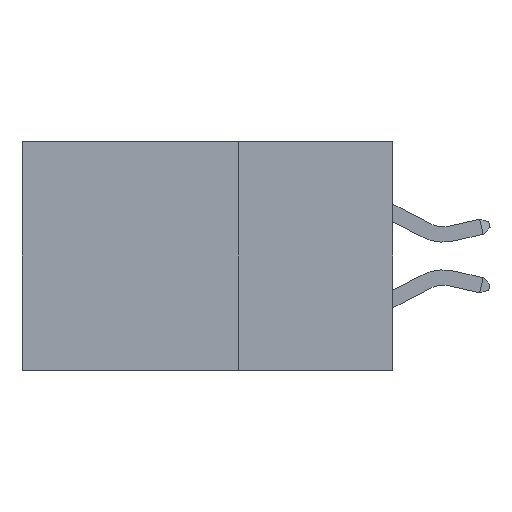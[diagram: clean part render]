
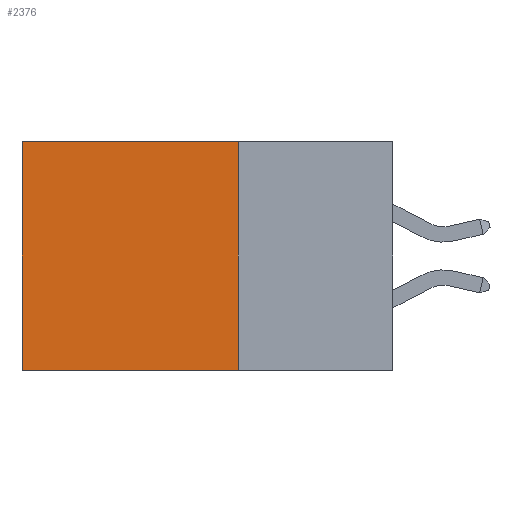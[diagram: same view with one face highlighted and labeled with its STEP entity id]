
A CAD part, left-side view. The second image highlights one B-rep face of the part: STEP entity #2376.
In plain terms, the highlighted planar face has unit normal (-1, 0, 0).
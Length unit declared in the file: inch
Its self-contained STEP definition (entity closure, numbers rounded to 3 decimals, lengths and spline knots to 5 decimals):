
#476 = VERTEX_POINT ( 'NONE', #19869 ) ;
#1830 = EDGE_CURVE ( 'NONE', #19514, #10616, #15404, .T. ) ;
#2038 = AXIS2_PLACEMENT_3D ( 'NONE', #9640, #19186, #17297 ) ;
#2376 = ADVANCED_FACE ( 'NONE', ( #4678 ), #13241, .F. ) ;
#2590 = ORIENTED_EDGE ( 'NONE', *, *, #21631, .T. ) ;
#2785 = CARTESIAN_POINT ( 'NONE',  ( 0.2875, 0.25, 0. ) ) ;
#2989 = CARTESIAN_POINT ( 'NONE',  ( 0.2875, 0.25, 0. ) ) ;
#4678 = FACE_OUTER_BOUND ( 'NONE', #10121, .T. ) ;
#5026 = VERTEX_POINT ( 'NONE', #10956 ) ;
#7851 = DIRECTION ( 'NONE',  ( 0., 1., 0. ) ) ;
#8581 = DIRECTION ( 'NONE',  ( 0., 0., -1. ) ) ;
#9120 = CARTESIAN_POINT ( 'NONE',  ( 0.2875, 0.25, -0.37 ) ) ;
#9324 = LINE ( 'NONE', #9120, #21638 ) ;
#9455 = EDGE_CURVE ( 'NONE', #10616, #476, #9324, .T. ) ;
#9640 = CARTESIAN_POINT ( 'NONE',  ( 0.2875, 0.25, 0. ) ) ;
#10121 = EDGE_LOOP ( 'NONE', ( #19588, #12713, #20958, #2590 ) ) ;
#10182 = CARTESIAN_POINT ( 'NONE',  ( 0.2875, 0.25, 0. ) ) ;
#10616 = VERTEX_POINT ( 'NONE', #12323 ) ;
#10956 = CARTESIAN_POINT ( 'NONE',  ( 0.2875, 0.6, 0. ) ) ;
#11323 = CARTESIAN_POINT ( 'NONE',  ( 0.2875, 0.6, 0. ) ) ;
#12323 = CARTESIAN_POINT ( 'NONE',  ( 0.2875, 0.25, -0.37 ) ) ;
#12662 = VECTOR ( 'NONE', #8581, 39.37008 ) ;
#12713 = ORIENTED_EDGE ( 'NONE', *, *, #9455, .F. ) ;
#13241 = PLANE ( 'NONE',  #2038 ) ;
#14236 = LINE ( 'NONE', #11323, #20996 ) ;
#15043 = DIRECTION ( 'NONE',  ( 0., 1., 0. ) ) ;
#15404 = LINE ( 'NONE', #2785, #12662 ) ;
#17297 = DIRECTION ( 'NONE',  ( 0., 0., -1. ) ) ;
#18915 = DIRECTION ( 'NONE',  ( 0., 0., -1. ) ) ;
#19186 = DIRECTION ( 'NONE',  ( 1., 0., 0. ) ) ;
#19514 = VERTEX_POINT ( 'NONE', #2989 ) ;
#19588 = ORIENTED_EDGE ( 'NONE', *, *, #20016, .T. ) ;
#19636 = LINE ( 'NONE', #10182, #20240 ) ;
#19869 = CARTESIAN_POINT ( 'NONE',  ( 0.2875, 0.6, -0.37 ) ) ;
#20016 = EDGE_CURVE ( 'NONE', #5026, #476, #14236, .T. ) ;
#20240 = VECTOR ( 'NONE', #7851, 39.37008 ) ;
#20958 = ORIENTED_EDGE ( 'NONE', *, *, #1830, .F. ) ;
#20996 = VECTOR ( 'NONE', #18915, 39.37008 ) ;
#21631 = EDGE_CURVE ( 'NONE', #19514, #5026, #19636, .T. ) ;
#21638 = VECTOR ( 'NONE', #15043, 39.37008 ) ;
